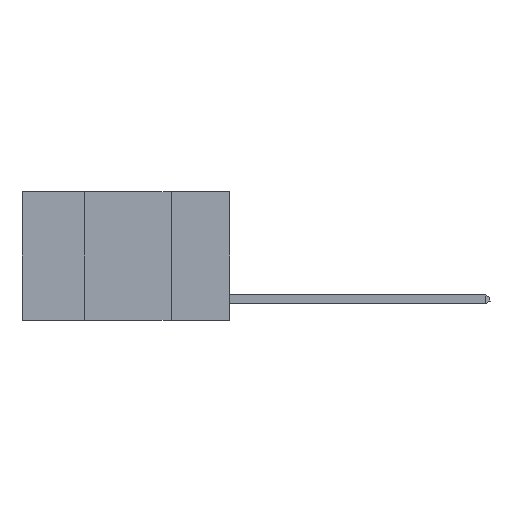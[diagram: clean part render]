
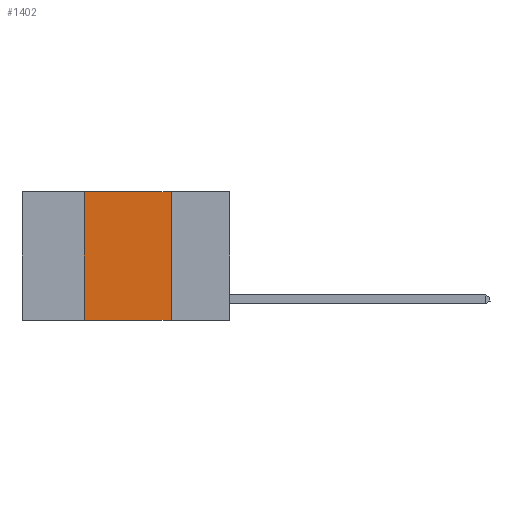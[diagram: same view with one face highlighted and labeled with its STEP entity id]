
A CAD part, left-side view. The second image highlights one B-rep face of the part: STEP entity #1402.
In plain terms, the highlighted planar face has unit normal (-1, 0, 0).
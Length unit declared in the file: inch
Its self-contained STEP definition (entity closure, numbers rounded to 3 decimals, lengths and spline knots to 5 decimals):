
#1402 = ADVANCED_FACE ( 'NONE', ( #8326 ), #12059, .F. ) ;
#1679 = ORIENTED_EDGE ( 'NONE', *, *, #6117, .T. ) ;
#1720 = ORIENTED_EDGE ( 'NONE', *, *, #2525, .F. ) ;
#2078 = CARTESIAN_POINT ( 'NONE',  ( 0., 0.6, -0.37 ) ) ;
#2082 = LINE ( 'NONE', #11164, #8097 ) ;
#2110 = LINE ( 'NONE', #13599, #14236 ) ;
#2525 = EDGE_CURVE ( 'NONE', #3627, #8176, #2082, .T. ) ;
#2712 = VERTEX_POINT ( 'NONE', #4506 ) ;
#3472 = VECTOR ( 'NONE', #5757, 39.37008 ) ;
#3627 = VERTEX_POINT ( 'NONE', #9689 ) ;
#4203 = DIRECTION ( 'NONE',  ( 0., 0., 1. ) ) ;
#4506 = CARTESIAN_POINT ( 'NONE',  ( 0., 0.17, -0.37 ) ) ;
#5491 = DIRECTION ( 'NONE',  ( 0., -1., 0. ) ) ;
#5651 = EDGE_LOOP ( 'NONE', ( #9249, #14428, #1720, #1679 ) ) ;
#5757 = DIRECTION ( 'NONE',  ( 0., 0., -1. ) ) ;
#6117 = EDGE_CURVE ( 'NONE', #3627, #2712, #6661, .T. ) ;
#6255 = DIRECTION ( 'NONE',  ( 0., 0., -1. ) ) ;
#6661 = LINE ( 'NONE', #2078, #9461 ) ;
#7038 = VERTEX_POINT ( 'NONE', #7447 ) ;
#7447 = CARTESIAN_POINT ( 'NONE',  ( 0., 0.17, 0. ) ) ;
#8097 = VECTOR ( 'NONE', #4203, 39.37008 ) ;
#8176 = VERTEX_POINT ( 'NONE', #13897 ) ;
#8326 = FACE_OUTER_BOUND ( 'NONE', #5651, .T. ) ;
#9249 = ORIENTED_EDGE ( 'NONE', *, *, #13426, .F. ) ;
#9461 = VECTOR ( 'NONE', #11532, 39.37008 ) ;
#9689 = CARTESIAN_POINT ( 'NONE',  ( 0., 0.42, -0.37 ) ) ;
#9761 = CARTESIAN_POINT ( 'NONE',  ( 0., 0.6, 0. ) ) ;
#9771 = LINE ( 'NONE', #12749, #3472 ) ;
#11164 = CARTESIAN_POINT ( 'NONE',  ( 0., 0.42, 0. ) ) ;
#11532 = DIRECTION ( 'NONE',  ( 0., -1., 0. ) ) ;
#12059 = PLANE ( 'NONE',  #12685 ) ;
#12685 = AXIS2_PLACEMENT_3D ( 'NONE', #9761, #13225, #6255 ) ;
#12749 = CARTESIAN_POINT ( 'NONE',  ( 0., 0.17, 0. ) ) ;
#13225 = DIRECTION ( 'NONE',  ( 1., 0., 0. ) ) ;
#13426 = EDGE_CURVE ( 'NONE', #7038, #2712, #9771, .T. ) ;
#13599 = CARTESIAN_POINT ( 'NONE',  ( 0., 0.6, 0. ) ) ;
#13897 = CARTESIAN_POINT ( 'NONE',  ( 0., 0.42, 0. ) ) ;
#14236 = VECTOR ( 'NONE', #5491, 39.37008 ) ;
#14428 = ORIENTED_EDGE ( 'NONE', *, *, #14831, .F. ) ;
#14831 = EDGE_CURVE ( 'NONE', #8176, #7038, #2110, .T. ) ;
